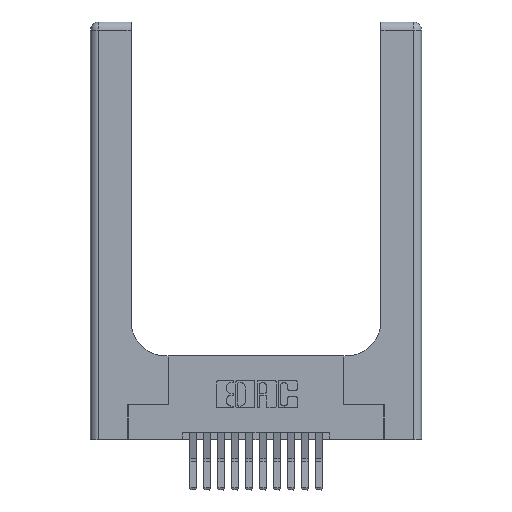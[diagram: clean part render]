
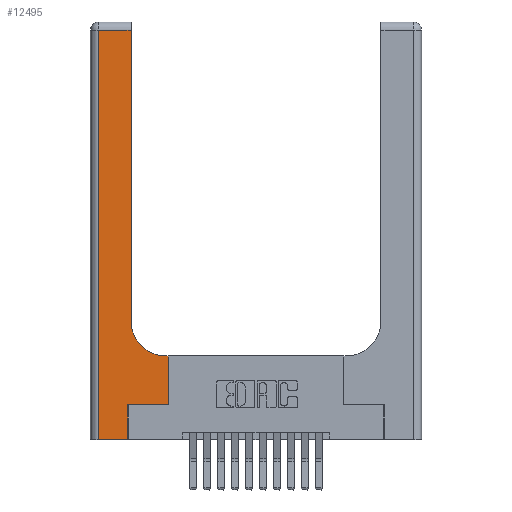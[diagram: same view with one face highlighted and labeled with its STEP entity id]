
A CAD part, top view. The second image highlights one B-rep face of the part: STEP entity #12495.
In plain terms, the highlighted planar face has unit normal (0, 0, 1).
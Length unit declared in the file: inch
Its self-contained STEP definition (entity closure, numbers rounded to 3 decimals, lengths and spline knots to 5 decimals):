
#5 = AXIS2_PLACEMENT_3D ( 'NONE', #5882, #11018, #9649 ) ;
#185 = ORIENTED_EDGE ( 'NONE', *, *, #7247, .T. ) ;
#687 = FACE_OUTER_BOUND ( 'NONE', #2987, .T. ) ;
#710 = CARTESIAN_POINT ( 'NONE',  ( 0.5585, 0.25, 0.37 ) ) ;
#1177 = LINE ( 'NONE', #13587, #6860 ) ;
#1374 = EDGE_CURVE ( 'NONE', #2039, #9674, #2344, .T. ) ;
#1403 = LINE ( 'NONE', #12989, #7906 ) ;
#1965 = CARTESIAN_POINT ( 'NONE',  ( 0.2915, 2.94, 0.37 ) ) ;
#2039 = VERTEX_POINT ( 'NONE', #1965 ) ;
#2281 = LINE ( 'NONE', #5998, #7956 ) ;
#2344 = LINE ( 'NONE', #5881, #6336 ) ;
#2403 = ORIENTED_EDGE ( 'NONE', *, *, #14937, .T. ) ;
#2554 = VECTOR ( 'NONE', #10350, 39.37008 ) ;
#2830 = ORIENTED_EDGE ( 'NONE', *, *, #5746, .T. ) ;
#2987 = EDGE_LOOP ( 'NONE', ( #185, #8646, #5461, #2830, #7478, #17333, #11601, #13271, #2403 ) ) ;
#3161 = CARTESIAN_POINT ( 'NONE',  ( 0.269, 0., 0.37 ) ) ;
#3498 = CARTESIAN_POINT ( 'NONE',  ( 0.5415, 0.6, 0.37 ) ) ;
#4506 = DIRECTION ( 'NONE',  ( -1., 0., 0. ) ) ;
#5297 = CARTESIAN_POINT ( 'NONE',  ( 0.269, 0., 0.37 ) ) ;
#5369 = CARTESIAN_POINT ( 'NONE',  ( 0.5585, 0.6, 0.37 ) ) ;
#5461 = ORIENTED_EDGE ( 'NONE', *, *, #17120, .T. ) ;
#5550 = VERTEX_POINT ( 'NONE', #16849 ) ;
#5746 = EDGE_CURVE ( 'NONE', #12266, #7655, #8875, .T. ) ;
#5881 = CARTESIAN_POINT ( 'NONE',  ( 0., 2.94, 0.37 ) ) ;
#5882 = CARTESIAN_POINT ( 'NONE',  ( 0.5415, 0.85, 0.37 ) ) ;
#5998 = CARTESIAN_POINT ( 'NONE',  ( 0.2915, 3., 0.37 ) ) ;
#6087 = LINE ( 'NONE', #710, #8829 ) ;
#6200 = VECTOR ( 'NONE', #10156, 39.37008 ) ;
#6336 = VECTOR ( 'NONE', #16645, 39.37008 ) ;
#6519 = VERTEX_POINT ( 'NONE', #16553 ) ;
#6576 = CARTESIAN_POINT ( 'NONE',  ( 0.269, 0.25, 0.37 ) ) ;
#6642 = EDGE_CURVE ( 'NONE', #5550, #7135, #6087, .T. ) ;
#6860 = VECTOR ( 'NONE', #15113, 39.37008 ) ;
#7135 = VERTEX_POINT ( 'NONE', #5369 ) ;
#7247 = EDGE_CURVE ( 'NONE', #6519, #2039, #2281, .T. ) ;
#7478 = ORIENTED_EDGE ( 'NONE', *, *, #15264, .T. ) ;
#7655 = VERTEX_POINT ( 'NONE', #3161 ) ;
#7906 = VECTOR ( 'NONE', #8935, 39.37008 ) ;
#7956 = VECTOR ( 'NONE', #11530, 39.37008 ) ;
#7977 = VERTEX_POINT ( 'NONE', #6576 ) ;
#8355 = CARTESIAN_POINT ( 'NONE',  ( 0.06, 2.94, 0.37 ) ) ;
#8413 = CARTESIAN_POINT ( 'NONE',  ( 0., 3., 0.37 ) ) ;
#8646 = ORIENTED_EDGE ( 'NONE', *, *, #1374, .T. ) ;
#8829 = VECTOR ( 'NONE', #13997, 39.37008 ) ;
#8875 = LINE ( 'NONE', #14119, #2554 ) ;
#8935 = DIRECTION ( 'NONE',  ( 0., -1., 0. ) ) ;
#9288 = EDGE_CURVE ( 'NONE', #7135, #15048, #1177, .T. ) ;
#9641 = VECTOR ( 'NONE', #16096, 39.37008 ) ;
#9649 = DIRECTION ( 'NONE',  ( 1., 0., 0. ) ) ;
#9674 = VERTEX_POINT ( 'NONE', #8355 ) ;
#10156 = DIRECTION ( 'NONE',  ( 1., 0., 0. ) ) ;
#10245 = AXIS2_PLACEMENT_3D ( 'NONE', #8413, #12590, #4506 ) ;
#10350 = DIRECTION ( 'NONE',  ( 1., 0., 0. ) ) ;
#10493 = LINE ( 'NONE', #5297, #9641 ) ;
#10619 = LINE ( 'NONE', #15559, #6200 ) ;
#10769 = PLANE ( 'NONE',  #10245 ) ;
#10780 = EDGE_CURVE ( 'NONE', #7977, #5550, #10619, .T. ) ;
#11018 = DIRECTION ( 'NONE',  ( 0., 0., -1. ) ) ;
#11530 = DIRECTION ( 'NONE',  ( 0., 1., 0. ) ) ;
#11601 = ORIENTED_EDGE ( 'NONE', *, *, #6642, .T. ) ;
#11805 = CARTESIAN_POINT ( 'NONE',  ( 0.06, 0., 0.37 ) ) ;
#12266 = VERTEX_POINT ( 'NONE', #11805 ) ;
#12495 = ADVANCED_FACE ( 'NONE', ( #687 ), #10769, .F. ) ;
#12590 = DIRECTION ( 'NONE',  ( 0., 0., -1. ) ) ;
#12817 = CIRCLE ( 'NONE', #5, 0.25 ) ;
#12989 = CARTESIAN_POINT ( 'NONE',  ( 0.06, 3., 0.37 ) ) ;
#13271 = ORIENTED_EDGE ( 'NONE', *, *, #9288, .T. ) ;
#13587 = CARTESIAN_POINT ( 'NONE',  ( 0.2915, 0.6, 0.37 ) ) ;
#13997 = DIRECTION ( 'NONE',  ( 0., 1., 0. ) ) ;
#14119 = CARTESIAN_POINT ( 'NONE',  ( 0., 0., 0.37 ) ) ;
#14937 = EDGE_CURVE ( 'NONE', #15048, #6519, #12817, .T. ) ;
#15048 = VERTEX_POINT ( 'NONE', #3498 ) ;
#15113 = DIRECTION ( 'NONE',  ( -1., 0., 0. ) ) ;
#15264 = EDGE_CURVE ( 'NONE', #7655, #7977, #10493, .T. ) ;
#15559 = CARTESIAN_POINT ( 'NONE',  ( 0.269, 0.25, 0.37 ) ) ;
#16096 = DIRECTION ( 'NONE',  ( 0., 1., 0. ) ) ;
#16553 = CARTESIAN_POINT ( 'NONE',  ( 0.2915, 0.85, 0.37 ) ) ;
#16645 = DIRECTION ( 'NONE',  ( -1., 0., 0. ) ) ;
#16849 = CARTESIAN_POINT ( 'NONE',  ( 0.5585, 0.25, 0.37 ) ) ;
#17120 = EDGE_CURVE ( 'NONE', #9674, #12266, #1403, .T. ) ;
#17333 = ORIENTED_EDGE ( 'NONE', *, *, #10780, .T. ) ;
